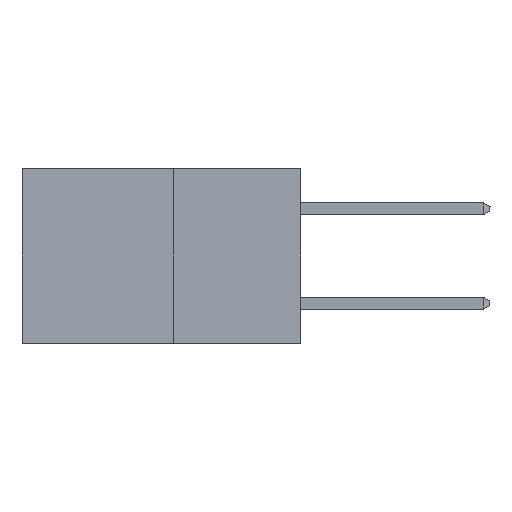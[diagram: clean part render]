
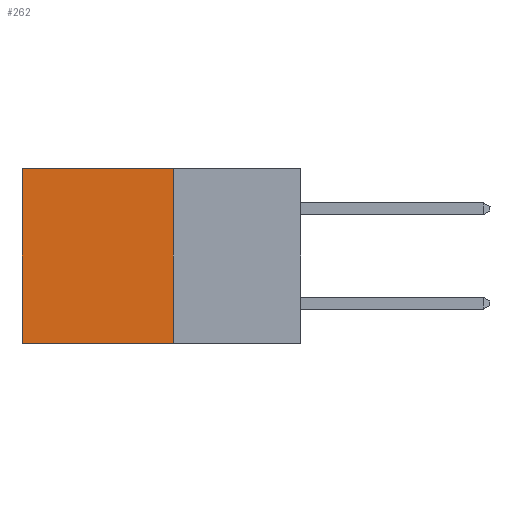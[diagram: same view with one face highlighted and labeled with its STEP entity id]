
A CAD part, left-side view. The second image highlights one B-rep face of the part: STEP entity #262.
In plain terms, the highlighted planar face has unit normal (-1, 0, 0).
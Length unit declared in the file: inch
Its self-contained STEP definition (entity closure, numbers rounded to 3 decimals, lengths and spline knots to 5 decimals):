
#7 = CARTESIAN_POINT ( 'NONE',  ( 0.277, 0.59, -0.37 ) ) ;
#262 = ADVANCED_FACE ( 'NONE', ( #3568 ), #8849, .F. ) ;
#272 = LINE ( 'NONE', #4883, #2410 ) ;
#1380 = ORIENTED_EDGE ( 'NONE', *, *, #9864, .T. ) ;
#1604 = ORIENTED_EDGE ( 'NONE', *, *, #6947, .T. ) ;
#2143 = VERTEX_POINT ( 'NONE', #7 ) ;
#2410 = VECTOR ( 'NONE', #3121, 39.37008 ) ;
#2635 = VERTEX_POINT ( 'NONE', #5628 ) ;
#2916 = VECTOR ( 'NONE', #8074, 39.37008 ) ;
#3075 = CARTESIAN_POINT ( 'NONE',  ( 0.277, 0.27, 0. ) ) ;
#3121 = DIRECTION ( 'NONE',  ( 0., 1., 0. ) ) ;
#3568 = FACE_OUTER_BOUND ( 'NONE', #4320, .T. ) ;
#4132 = EDGE_CURVE ( 'NONE', #9939, #2143, #272, .T. ) ;
#4146 = EDGE_CURVE ( 'NONE', #6402, #9939, #4740, .T. ) ;
#4320 = EDGE_LOOP ( 'NONE', ( #1604, #4886, #4465, #1380 ) ) ;
#4465 = ORIENTED_EDGE ( 'NONE', *, *, #4146, .F. ) ;
#4503 = CARTESIAN_POINT ( 'NONE',  ( 0.277, 0.27, -0.37 ) ) ;
#4740 = LINE ( 'NONE', #7300, #8964 ) ;
#4883 = CARTESIAN_POINT ( 'NONE',  ( 0.277, 0.27, -0.37 ) ) ;
#4886 = ORIENTED_EDGE ( 'NONE', *, *, #4132, .F. ) ;
#5357 = DIRECTION ( 'NONE',  ( 1., 0., 0. ) ) ;
#5586 = CARTESIAN_POINT ( 'NONE',  ( 0.277, 0.27, -0.37 ) ) ;
#5628 = CARTESIAN_POINT ( 'NONE',  ( 0.277, 0.59, 0. ) ) ;
#5783 = AXIS2_PLACEMENT_3D ( 'NONE', #5586, #5357, #10858 ) ;
#6249 = LINE ( 'NONE', #7763, #8222 ) ;
#6402 = VERTEX_POINT ( 'NONE', #3075 ) ;
#6947 = EDGE_CURVE ( 'NONE', #2635, #2143, #9160, .T. ) ;
#7221 = CARTESIAN_POINT ( 'NONE',  ( 0.277, 0.59, -0.37 ) ) ;
#7300 = CARTESIAN_POINT ( 'NONE',  ( 0.277, 0.27, -0.37 ) ) ;
#7763 = CARTESIAN_POINT ( 'NONE',  ( 0.277, 0.27, 0. ) ) ;
#8074 = DIRECTION ( 'NONE',  ( 0., 0., -1. ) ) ;
#8222 = VECTOR ( 'NONE', #11089, 39.37008 ) ;
#8849 = PLANE ( 'NONE',  #5783 ) ;
#8964 = VECTOR ( 'NONE', #9884, 39.37008 ) ;
#9160 = LINE ( 'NONE', #7221, #2916 ) ;
#9864 = EDGE_CURVE ( 'NONE', #6402, #2635, #6249, .T. ) ;
#9884 = DIRECTION ( 'NONE',  ( 0., 0., -1. ) ) ;
#9939 = VERTEX_POINT ( 'NONE', #4503 ) ;
#10858 = DIRECTION ( 'NONE',  ( 0., 0., -1. ) ) ;
#11089 = DIRECTION ( 'NONE',  ( 0., 1., 0. ) ) ;
